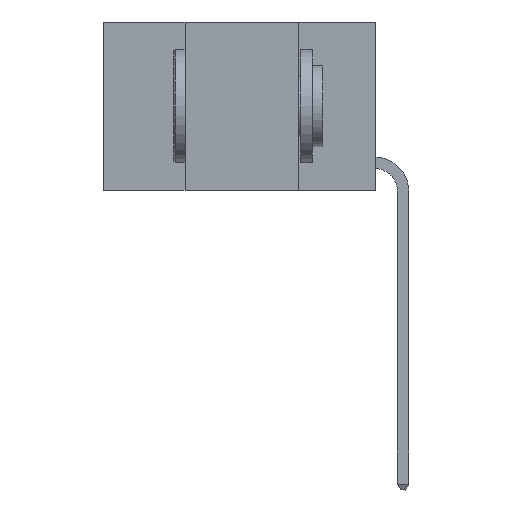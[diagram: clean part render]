
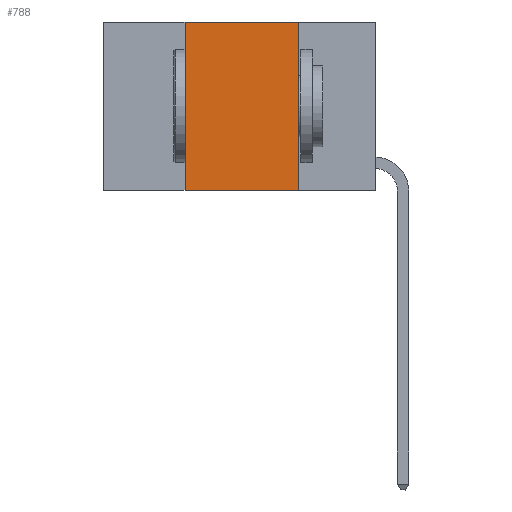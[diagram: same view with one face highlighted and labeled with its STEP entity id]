
A CAD part, left-side view. The second image highlights one B-rep face of the part: STEP entity #788.
In plain terms, the highlighted planar face has unit normal (-1, 0, 0).
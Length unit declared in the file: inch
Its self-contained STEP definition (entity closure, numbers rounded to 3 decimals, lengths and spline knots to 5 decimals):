
#173 = VECTOR ( 'NONE', #8538, 39.37008 ) ;
#788 = ADVANCED_FACE ( 'NONE', ( #9650 ), #9374, .F. ) ;
#1545 = EDGE_CURVE ( 'NONE', #8630, #4236, #10056, .T. ) ;
#1579 = EDGE_CURVE ( 'NONE', #8630, #5321, #4561, .T. ) ;
#1733 = VECTOR ( 'NONE', #8243, 39.37008 ) ;
#2687 = CARTESIAN_POINT ( 'NONE',  ( 0., 0.6, 0. ) ) ;
#4236 = VERTEX_POINT ( 'NONE', #12240 ) ;
#4561 = LINE ( 'NONE', #8839, #1733 ) ;
#4806 = VECTOR ( 'NONE', #12497, 39.37008 ) ;
#4971 = EDGE_LOOP ( 'NONE', ( #7917, #8088, #8110, #8146 ) ) ;
#5321 = VERTEX_POINT ( 'NONE', #7960 ) ;
#5763 = VECTOR ( 'NONE', #5853, 39.37008 ) ;
#5853 = DIRECTION ( 'NONE',  ( 0., -1., 0. ) ) ;
#7917 = ORIENTED_EDGE ( 'NONE', *, *, #10979, .F. ) ;
#7960 = CARTESIAN_POINT ( 'NONE',  ( 0., 0.17, -0.37 ) ) ;
#8088 = ORIENTED_EDGE ( 'NONE', *, *, #10853, .F. ) ;
#8110 = ORIENTED_EDGE ( 'NONE', *, *, #1545, .F. ) ;
#8146 = ORIENTED_EDGE ( 'NONE', *, *, #1579, .T. ) ;
#8243 = DIRECTION ( 'NONE',  ( 0., -1., 0. ) ) ;
#8326 = LINE ( 'NONE', #2687, #5763 ) ;
#8538 = DIRECTION ( 'NONE',  ( 0., 0., 1. ) ) ;
#8620 = CARTESIAN_POINT ( 'NONE',  ( 0., 0.42, 0. ) ) ;
#8630 = VERTEX_POINT ( 'NONE', #11197 ) ;
#8839 = CARTESIAN_POINT ( 'NONE',  ( 0., 0.6, -0.37 ) ) ;
#9374 = PLANE ( 'NONE',  #12140 ) ;
#9415 = DIRECTION ( 'NONE',  ( 0., 0., -1. ) ) ;
#9444 = DIRECTION ( 'NONE',  ( 1., 0., 0. ) ) ;
#9650 = FACE_OUTER_BOUND ( 'NONE', #4971, .T. ) ;
#9799 = CARTESIAN_POINT ( 'NONE',  ( 0., 0.17, 0. ) ) ;
#9848 = CARTESIAN_POINT ( 'NONE',  ( 0., 0.6, 0. ) ) ;
#10056 = LINE ( 'NONE', #8620, #173 ) ;
#10699 = CARTESIAN_POINT ( 'NONE',  ( 0., 0.17, 0. ) ) ;
#10853 = EDGE_CURVE ( 'NONE', #4236, #12764, #8326, .T. ) ;
#10979 = EDGE_CURVE ( 'NONE', #12764, #5321, #12380, .T. ) ;
#11197 = CARTESIAN_POINT ( 'NONE',  ( 0., 0.42, -0.37 ) ) ;
#12140 = AXIS2_PLACEMENT_3D ( 'NONE', #9848, #9444, #9415 ) ;
#12240 = CARTESIAN_POINT ( 'NONE',  ( 0., 0.42, 0. ) ) ;
#12380 = LINE ( 'NONE', #10699, #4806 ) ;
#12497 = DIRECTION ( 'NONE',  ( 0., 0., -1. ) ) ;
#12764 = VERTEX_POINT ( 'NONE', #9799 ) ;
